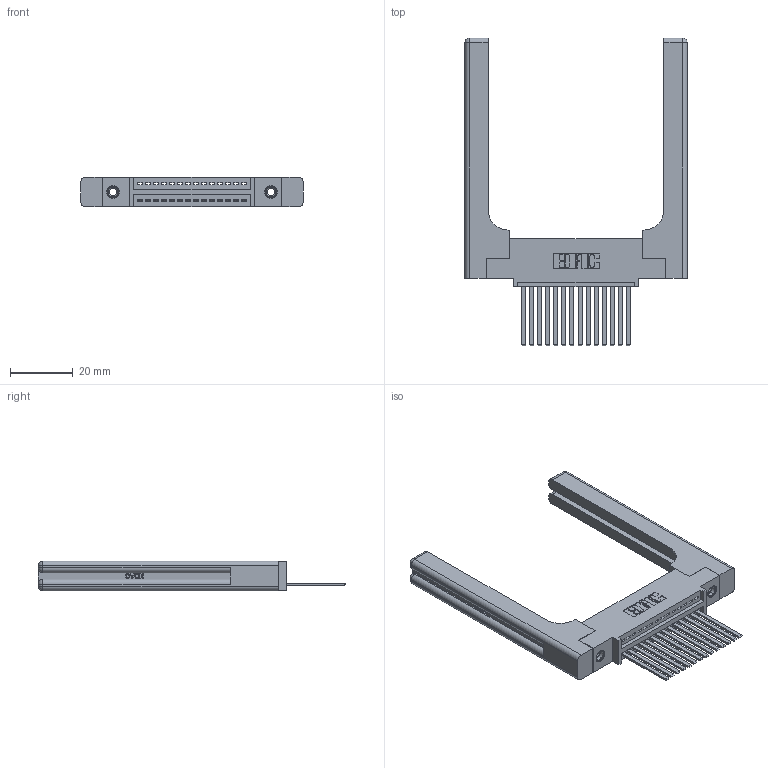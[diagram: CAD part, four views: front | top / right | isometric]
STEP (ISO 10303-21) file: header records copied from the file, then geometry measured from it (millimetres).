
FILE_DESCRIPTION (( 'STEP AP203' ), '1' );
FILE_NAME ('345-014-544-458.STEP', '2019-10-04T11:17:58', ( '' ), ( '' ), 'SwSTEP 2.0', 'SolidWorks 2016', '' );
FILE_SCHEMA (( 'CONFIG_CONTROL_DESIGN' ));
Length unit declared in the file: inch
Products named in the file (5): 345-220-058_345-220-058; 345-250-001_345-250-001-102; 345-292-001_345-293-144; 345-014-544-458; 345 Part_0.110 Offset - 0.156 Dia-TH
Assembly tree (19 placements, depth 2):
  345-014-544-458
    345 Part_0.110 Offset - 0.156 Dia-TH
    345-292-001_345-293-144  x14
    345-250-001_345-250-001-102  x2
    345-220-058_345-220-058  x2
Bounding box: 70.59 x 97.71 x 9.4 mm (x, y, z)
Volume: 15068.8 mm3; surface area: 14216.3 mm2
Topology: 19 solids, 19 shells, 1114 faces, 3231 edges, 2114 vertices
Faces by surface type: plane 736, cylinder 318, bspline 36, cone 12, sphere 8, torus 4
Entity records: 19436 total; most frequent: CARTESIAN_POINT 4339, ORIENTED_EDGE 3084, DIRECTION 2774, EDGE_CURVE 1542, VECTOR 1266, LINE 1266, VERTEX_POINT 1018, AXIS2_PLACEMENT_3D 754
